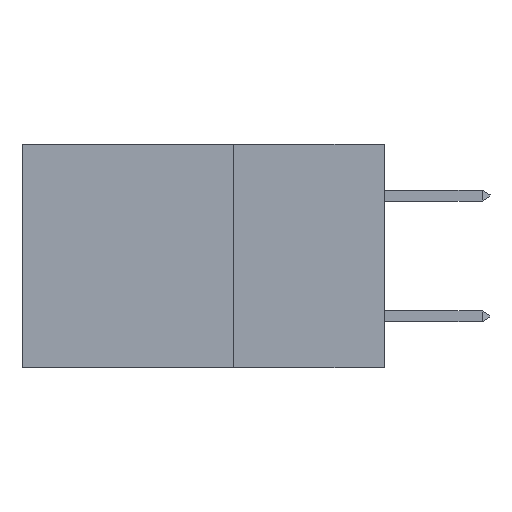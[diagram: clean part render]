
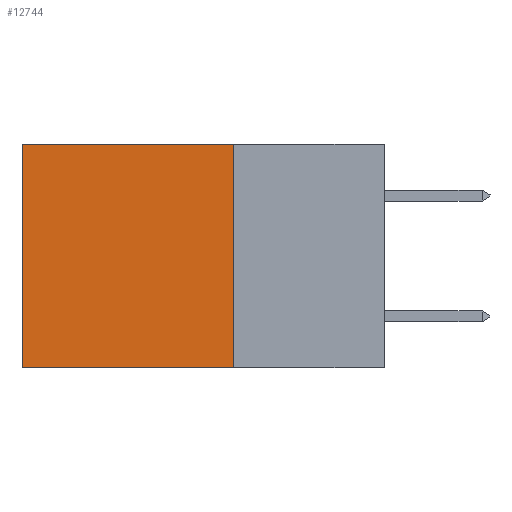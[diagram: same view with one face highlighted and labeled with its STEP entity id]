
A CAD part, left-side view. The second image highlights one B-rep face of the part: STEP entity #12744.
In plain terms, the highlighted planar face has unit normal (-1, 0, 0).
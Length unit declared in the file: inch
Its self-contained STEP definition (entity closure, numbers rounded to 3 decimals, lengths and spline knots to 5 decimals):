
#365 = CARTESIAN_POINT ( 'NONE',  ( 0.2875, 0.6, -0.37 ) ) ;
#368 = PLANE ( 'NONE',  #2115 ) ;
#1383 = DIRECTION ( 'NONE',  ( 1., 0., 0. ) ) ;
#1432 = DIRECTION ( 'NONE',  ( 0., 0., -1. ) ) ;
#1919 = EDGE_CURVE ( 'NONE', #9027, #6380, #2091, .T. ) ;
#2091 = LINE ( 'NONE', #8154, #4735 ) ;
#2115 = AXIS2_PLACEMENT_3D ( 'NONE', #7344, #1383, #10309 ) ;
#3743 = VERTEX_POINT ( 'NONE', #6452 ) ;
#4568 = DIRECTION ( 'NONE',  ( 0., 1., 0. ) ) ;
#4735 = VECTOR ( 'NONE', #10230, 39.37008 ) ;
#4969 = EDGE_CURVE ( 'NONE', #3743, #9027, #6796, .T. ) ;
#5197 = ORIENTED_EDGE ( 'NONE', *, *, #1919, .T. ) ;
#5404 = VECTOR ( 'NONE', #12506, 39.37008 ) ;
#5438 = CARTESIAN_POINT ( 'NONE',  ( 0.2875, 0.6, 0. ) ) ;
#5470 = CARTESIAN_POINT ( 'NONE',  ( 0.2875, 0.25, 0. ) ) ;
#5927 = ORIENTED_EDGE ( 'NONE', *, *, #9852, .F. ) ;
#6179 = LINE ( 'NONE', #10457, #5404 ) ;
#6380 = VERTEX_POINT ( 'NONE', #365 ) ;
#6452 = CARTESIAN_POINT ( 'NONE',  ( 0.2875, 0.25, 0. ) ) ;
#6796 = LINE ( 'NONE', #5470, #8676 ) ;
#6980 = VECTOR ( 'NONE', #1432, 39.37008 ) ;
#7279 = ORIENTED_EDGE ( 'NONE', *, *, #4969, .T. ) ;
#7344 = CARTESIAN_POINT ( 'NONE',  ( 0.2875, 0.25, 0. ) ) ;
#7408 = FACE_OUTER_BOUND ( 'NONE', #10059, .T. ) ;
#8154 = CARTESIAN_POINT ( 'NONE',  ( 0.2875, 0.6, 0. ) ) ;
#8317 = CARTESIAN_POINT ( 'NONE',  ( 0.2875, 0.25, 0. ) ) ;
#8482 = VERTEX_POINT ( 'NONE', #11755 ) ;
#8676 = VECTOR ( 'NONE', #4568, 39.37008 ) ;
#9027 = VERTEX_POINT ( 'NONE', #5438 ) ;
#9209 = ORIENTED_EDGE ( 'NONE', *, *, #11779, .F. ) ;
#9637 = LINE ( 'NONE', #8317, #6980 ) ;
#9852 = EDGE_CURVE ( 'NONE', #3743, #8482, #9637, .T. ) ;
#10059 = EDGE_LOOP ( 'NONE', ( #5197, #9209, #5927, #7279 ) ) ;
#10230 = DIRECTION ( 'NONE',  ( 0., 0., -1. ) ) ;
#10309 = DIRECTION ( 'NONE',  ( 0., 0., -1. ) ) ;
#10457 = CARTESIAN_POINT ( 'NONE',  ( 0.2875, 0.25, -0.37 ) ) ;
#11755 = CARTESIAN_POINT ( 'NONE',  ( 0.2875, 0.25, -0.37 ) ) ;
#11779 = EDGE_CURVE ( 'NONE', #8482, #6380, #6179, .T. ) ;
#12506 = DIRECTION ( 'NONE',  ( 0., 1., 0. ) ) ;
#12744 = ADVANCED_FACE ( 'NONE', ( #7408 ), #368, .F. ) ;
